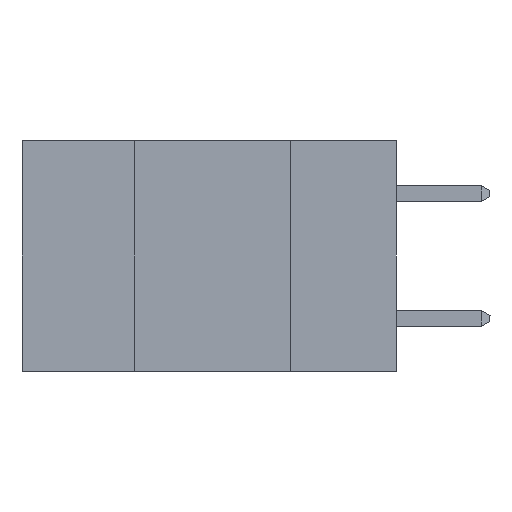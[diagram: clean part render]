
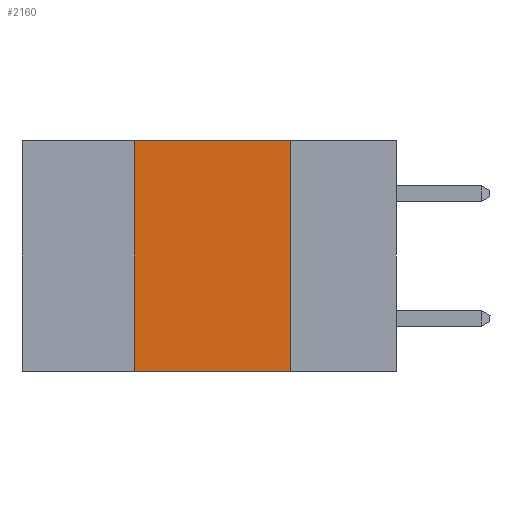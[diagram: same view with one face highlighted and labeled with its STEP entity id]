
A CAD part, left-side view. The second image highlights one B-rep face of the part: STEP entity #2160.
In plain terms, the highlighted planar face has unit normal (-1, 0, 0).
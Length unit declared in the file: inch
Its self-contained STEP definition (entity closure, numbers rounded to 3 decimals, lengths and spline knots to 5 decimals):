
#438 = CARTESIAN_POINT ( 'NONE',  ( 0., 0.42, -0.37 ) ) ;
#1043 = CARTESIAN_POINT ( 'NONE',  ( 0., 0.6, 0. ) ) ;
#1187 = VECTOR ( 'NONE', #2116, 39.37008 ) ;
#1548 = VERTEX_POINT ( 'NONE', #9806 ) ;
#1689 = DIRECTION ( 'NONE',  ( 0., 0., -1. ) ) ;
#1698 = EDGE_LOOP ( 'NONE', ( #8461, #1976, #9432, #2656 ) ) ;
#1976 = ORIENTED_EDGE ( 'NONE', *, *, #11355, .F. ) ;
#2116 = DIRECTION ( 'NONE',  ( 0., -1., 0. ) ) ;
#2135 = CARTESIAN_POINT ( 'NONE',  ( 0., 0.6, 0. ) ) ;
#2160 = ADVANCED_FACE ( 'NONE', ( #9209 ), #6967, .F. ) ;
#2350 = DIRECTION ( 'NONE',  ( 0., 0., -1. ) ) ;
#2656 = ORIENTED_EDGE ( 'NONE', *, *, #4469, .T. ) ;
#2833 = CARTESIAN_POINT ( 'NONE',  ( 0., 0.17, 0. ) ) ;
#3833 = LINE ( 'NONE', #1043, #1187 ) ;
#4159 = VECTOR ( 'NONE', #8008, 39.37008 ) ;
#4469 = EDGE_CURVE ( 'NONE', #1548, #9926, #9430, .T. ) ;
#4471 = LINE ( 'NONE', #438, #4159 ) ;
#4488 = CARTESIAN_POINT ( 'NONE',  ( 0., 0.42, 0. ) ) ;
#5495 = CARTESIAN_POINT ( 'NONE',  ( 0., 0.17, -0.37 ) ) ;
#5719 = EDGE_CURVE ( 'NONE', #7309, #9926, #10060, .T. ) ;
#6726 = DIRECTION ( 'NONE',  ( 1., 0., 0. ) ) ;
#6937 = CARTESIAN_POINT ( 'NONE',  ( 0., 0.6, -0.37 ) ) ;
#6967 = PLANE ( 'NONE',  #8459 ) ;
#7309 = VERTEX_POINT ( 'NONE', #2833 ) ;
#7812 = VECTOR ( 'NONE', #1689, 39.37008 ) ;
#7817 = DIRECTION ( 'NONE',  ( 0., -1., 0. ) ) ;
#8008 = DIRECTION ( 'NONE',  ( 0., 0., 1. ) ) ;
#8035 = EDGE_CURVE ( 'NONE', #1548, #8922, #4471, .T. ) ;
#8459 = AXIS2_PLACEMENT_3D ( 'NONE', #2135, #6726, #2350 ) ;
#8461 = ORIENTED_EDGE ( 'NONE', *, *, #5719, .F. ) ;
#8922 = VERTEX_POINT ( 'NONE', #4488 ) ;
#9209 = FACE_OUTER_BOUND ( 'NONE', #1698, .T. ) ;
#9430 = LINE ( 'NONE', #6937, #10207 ) ;
#9432 = ORIENTED_EDGE ( 'NONE', *, *, #8035, .F. ) ;
#9806 = CARTESIAN_POINT ( 'NONE',  ( 0., 0.42, -0.37 ) ) ;
#9926 = VERTEX_POINT ( 'NONE', #5495 ) ;
#10060 = LINE ( 'NONE', #10546, #7812 ) ;
#10207 = VECTOR ( 'NONE', #7817, 39.37008 ) ;
#10546 = CARTESIAN_POINT ( 'NONE',  ( 0., 0.17, -0.37 ) ) ;
#11355 = EDGE_CURVE ( 'NONE', #8922, #7309, #3833, .T. ) ;
